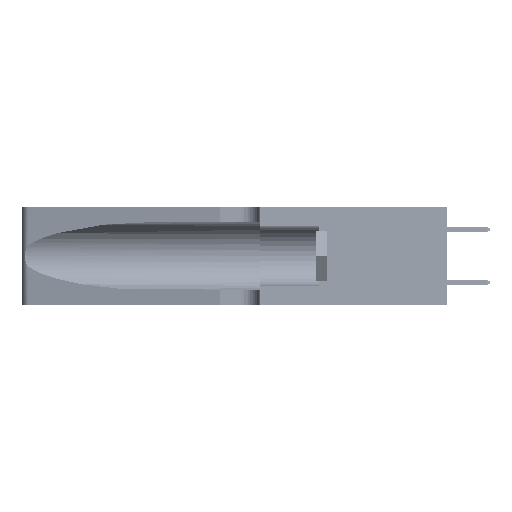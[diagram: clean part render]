
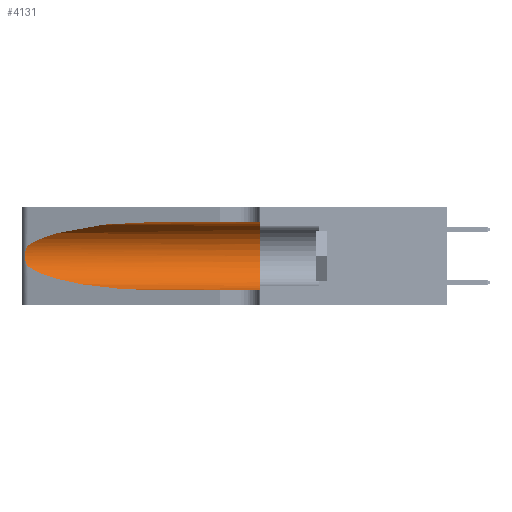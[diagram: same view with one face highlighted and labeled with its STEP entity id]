
A CAD part, left-side view. The second image highlights one B-rep face of the part: STEP entity #4131.
In plain terms, the highlighted cylindrical face has radius 3.308 mm (diameter 6.617 mm), a partial arc.
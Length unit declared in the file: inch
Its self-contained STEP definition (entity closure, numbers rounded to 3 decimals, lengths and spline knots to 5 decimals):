
#609 = CARTESIAN_POINT ( 'NONE',  ( 0.25789, 1.23486, 0.15765 ) ) ;
#864 = EDGE_LOOP ( 'NONE', ( #26620, #38275, #20136, #27559, #37536, #15601 ) ) ;
#1025 = DIRECTION ( 'NONE',  ( 0., -1., 0. ) ) ;
#1108 = CARTESIAN_POINT ( 'NONE',  ( 0.25487, 1.22718, 0.22369 ) ) ;
#2899 = CARTESIAN_POINT ( 'NONE',  ( 0.1305, 0.35, 0.05475 ) ) ;
#3648 = EDGE_CURVE ( 'NONE', #51826, #17451, #29248, .T. ) ;
#3927 = DIRECTION ( 'NONE',  ( 0., -1., 0. ) ) ;
#4131 = ADVANCED_FACE ( 'NONE', ( #26575 ), #47723, .F. ) ;
#4859 = CARTESIAN_POINT ( 'NONE',  ( 0.25555, 1.22993, 0.14849 ) ) ;
#4996 = CARTESIAN_POINT ( 'NONE',  ( 0.2373, 1.15595, 0.28018 ) ) ;
#5836 = DIRECTION ( 'NONE',  ( 0., 1., 0. ) ) ;
#10285 = CARTESIAN_POINT ( 'NONE',  ( 0.18966, 0.96281, 0.05475 ) ) ;
#10323 = AXIS2_PLACEMENT_3D ( 'NONE', #31308, #5836, #35558 ) ;
#10532 = CARTESIAN_POINT ( 'NONE',  ( 0.25487, 1.22718, 0.14631 ) ) ;
#11774 = CARTESIAN_POINT ( 'NONE',  ( 0.1305, 0.72297, 0.05475 ) ) ;
#13280 = CARTESIAN_POINT ( 'NONE',  ( 0.25787, 1.23484, 0.2124 ) ) ;
#13321 = EDGE_CURVE ( 'NONE', #33016, #51826, #49742, .T. ) ;
#13708 = LINE ( 'NONE', #27164, #34927 ) ;
#14575 = CARTESIAN_POINT ( 'NONE',  ( 0.1305, 0.72297, 0.05475 ) ) ;
#15601 = ORIENTED_EDGE ( 'NONE', *, *, #33670, .F. ) ;
#16379 = EDGE_CURVE ( 'NONE', #44800, #33016, #39957, .T. ) ;
#16603 = CARTESIAN_POINT ( 'NONE',  ( 0.1305, 1.61858, 0.185 ) ) ;
#17360 = CARTESIAN_POINT ( 'NONE',  ( 0.25487, 1.22718, 0.22369 ) ) ;
#17451 = VERTEX_POINT ( 'NONE', #2899 ) ;
#17539 = CARTESIAN_POINT ( 'NONE',  ( 0.26018, 1.23835, 0.19895 ) ) ;
#18599 = CARTESIAN_POINT ( 'NONE',  ( 0.2373, 1.15595, 0.08982 ) ) ;
#19043 = EDGE_CURVE ( 'NONE', #44354, #44800, #20198, .T. ) ;
#19395 = CIRCLE ( 'NONE', #10323, 0.13025 ) ;
#20136 = ORIENTED_EDGE ( 'NONE', *, *, #13321, .T. ) ;
#20198 =( BOUNDED_CURVE ( )  B_SPLINE_CURVE ( 3, ( #26224, #51487, #4996, #34721 ),
 .UNSPECIFIED., .F., .T. ) 
 B_SPLINE_CURVE_WITH_KNOTS ( ( 4, 4 ),
 ( 1.5708, 2.84003 ),
 .UNSPECIFIED. ) 
 CURVE ( )  GEOMETRIC_REPRESENTATION_ITEM ( )  RATIONAL_B_SPLINE_CURVE ( ( 1., 0.87, 0.87, 1. ) ) 
 REPRESENTATION_ITEM ( '' )  );
#21767 = CARTESIAN_POINT ( 'NONE',  ( 0.26075, 1.23896, 0.178 ) ) ;
#25127 = VERTEX_POINT ( 'NONE', #47708 ) ;
#26090 = CARTESIAN_POINT ( 'NONE',  ( 0.25856, 1.23593, 0.16098 ) ) ;
#26224 = CARTESIAN_POINT ( 'NONE',  ( 0.1305, 0.72297, 0.31525 ) ) ;
#26575 = FACE_OUTER_BOUND ( 'NONE', #864, .T. ) ;
#26620 = ORIENTED_EDGE ( 'NONE', *, *, #19043, .T. ) ;
#27164 = CARTESIAN_POINT ( 'NONE',  ( 0.1305, 1.61858, 0.31525 ) ) ;
#27559 = ORIENTED_EDGE ( 'NONE', *, *, #3648, .T. ) ;
#29209 = DIRECTION ( 'NONE',  ( 0., 0., -1. ) ) ;
#29248 = LINE ( 'NONE', #51791, #50385 ) ;
#30307 = CARTESIAN_POINT ( 'NONE',  ( 0.25639, 1.23186, 0.15144 ) ) ;
#31308 = CARTESIAN_POINT ( 'NONE',  ( 0.1305, 0.35, 0.185 ) ) ;
#31419 = DIRECTION ( 'NONE',  ( 0., -1., 0. ) ) ;
#32963 = EDGE_CURVE ( 'NONE', #25127, #17451, #19395, .T. ) ;
#33016 = VERTEX_POINT ( 'NONE', #10532 ) ;
#33670 = EDGE_CURVE ( 'NONE', #44354, #25127, #13708, .T. ) ;
#34408 = CARTESIAN_POINT ( 'NONE',  ( 0.25555, 1.22994, 0.2215 ) ) ;
#34600 = CARTESIAN_POINT ( 'NONE',  ( 0.25487, 1.22718, 0.14631 ) ) ;
#34721 = CARTESIAN_POINT ( 'NONE',  ( 0.25487, 1.22718, 0.22369 ) ) ;
#34927 = VECTOR ( 'NONE', #31419, 39.37008 ) ;
#35558 = DIRECTION ( 'NONE',  ( 0., 0., 1. ) ) ;
#36446 = CARTESIAN_POINT ( 'NONE',  ( 0.1305, 0.72297, 0.31525 ) ) ;
#37415 = AXIS2_PLACEMENT_3D ( 'NONE', #16603, #3927, #29209 ) ;
#37536 = ORIENTED_EDGE ( 'NONE', *, *, #32963, .F. ) ;
#38275 = ORIENTED_EDGE ( 'NONE', *, *, #16379, .T. ) ;
#38649 = CARTESIAN_POINT ( 'NONE',  ( 0.25639, 1.23184, 0.21858 ) ) ;
#39957 = B_SPLINE_CURVE_WITH_KNOTS ( 'NONE', 3,
 ( #17360, #34408, #38649, #13280, #42895, #17539, #47148, #21767, #51360, #26090, #609, #30307, #4859, #34600 ),
 .UNSPECIFIED., .F., .F.,
 ( 4, 2, 2, 2, 2, 2, 4 ),
 ( 0., 0.00027, 0.00053, 0.00107, 0.0016, 0.00187, 0.00214 ),
 .UNSPECIFIED. ) ;
#42895 = CARTESIAN_POINT ( 'NONE',  ( 0.25854, 1.2359, 0.20912 ) ) ;
#44354 = VERTEX_POINT ( 'NONE', #36446 ) ;
#44800 = VERTEX_POINT ( 'NONE', #1108 ) ;
#47148 = CARTESIAN_POINT ( 'NONE',  ( 0.26075, 1.23896, 0.19203 ) ) ;
#47708 = CARTESIAN_POINT ( 'NONE',  ( 0.1305, 0.35, 0.31525 ) ) ;
#47723 = CYLINDRICAL_SURFACE ( 'NONE', #37415, 0.13025 ) ;
#49742 =( BOUNDED_CURVE ( )  B_SPLINE_CURVE ( 3, ( #52456, #18599, #10285, #14575 ),
 .UNSPECIFIED., .F., .F. ) 
 B_SPLINE_CURVE_WITH_KNOTS ( ( 4, 4 ),
 ( 3.44316, 4.71239 ),
 .UNSPECIFIED. ) 
 CURVE ( )  GEOMETRIC_REPRESENTATION_ITEM ( )  RATIONAL_B_SPLINE_CURVE ( ( 1., 0.87, 0.87, 1. ) ) 
 REPRESENTATION_ITEM ( '' )  );
#50385 = VECTOR ( 'NONE', #1025, 39.37008 ) ;
#51360 = CARTESIAN_POINT ( 'NONE',  ( 0.26017, 1.23833, 0.17102 ) ) ;
#51487 = CARTESIAN_POINT ( 'NONE',  ( 0.18966, 0.96281, 0.31525 ) ) ;
#51791 = CARTESIAN_POINT ( 'NONE',  ( 0.1305, 1.61858, 0.05475 ) ) ;
#51826 = VERTEX_POINT ( 'NONE', #11774 ) ;
#52456 = CARTESIAN_POINT ( 'NONE',  ( 0.25487, 1.22718, 0.14631 ) ) ;
